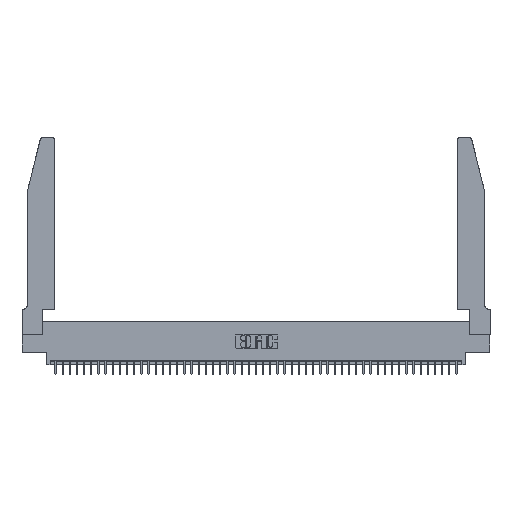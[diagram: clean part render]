
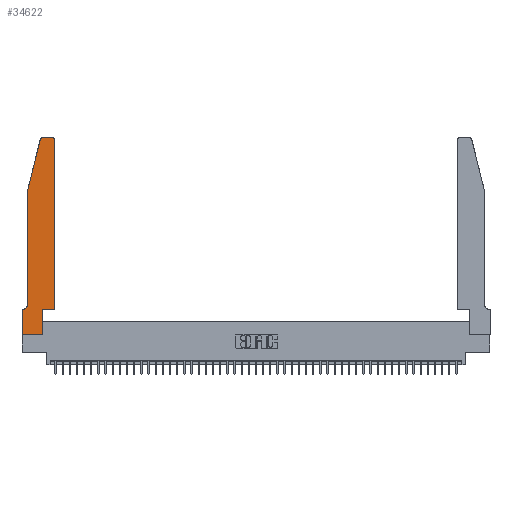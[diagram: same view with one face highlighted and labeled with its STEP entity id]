
A CAD part, top view. The second image highlights one B-rep face of the part: STEP entity #34622.
In plain terms, the highlighted planar face has unit normal (0, 0, 1).
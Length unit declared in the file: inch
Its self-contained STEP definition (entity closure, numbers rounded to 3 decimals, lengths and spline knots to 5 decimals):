
#530 = CARTESIAN_POINT ( 'NONE',  ( 0., 0.35, 0.37 ) ) ;
#876 = VERTEX_POINT ( 'NONE', #14309 ) ;
#877 = DIRECTION ( 'NONE',  ( 0., 1., 0. ) ) ;
#885 = ORIENTED_EDGE ( 'NONE', *, *, #32314, .T. ) ;
#1425 = CARTESIAN_POINT ( 'NONE',  ( 0.0755, 2., 0.37 ) ) ;
#1626 = DIRECTION ( 'NONE',  ( 1., 0., 0. ) ) ;
#1682 = CARTESIAN_POINT ( 'NONE',  ( 0.0755, 2., 0.37 ) ) ;
#1829 = ORIENTED_EDGE ( 'NONE', *, *, #39078, .T. ) ;
#3073 = VERTEX_POINT ( 'NONE', #26422 ) ;
#3277 = VECTOR ( 'NONE', #16940, 39.37008 ) ;
#4284 = CARTESIAN_POINT ( 'NONE',  ( 0.4505, 0.35, 0.37 ) ) ;
#4402 = CARTESIAN_POINT ( 'NONE',  ( 0., 0.35, 0.37 ) ) ;
#5119 = FACE_OUTER_BOUND ( 'NONE', #25854, .T. ) ;
#5715 = VECTOR ( 'NONE', #12567, 39.37008 ) ;
#6719 = CIRCLE ( 'NONE', #35302, 0.03 ) ;
#7092 = CARTESIAN_POINT ( 'NONE',  ( 0.0755, 2., 0.37 ) ) ;
#8177 = LINE ( 'NONE', #20017, #19759 ) ;
#8626 = VERTEX_POINT ( 'NONE', #4402 ) ;
#9294 = DIRECTION ( 'NONE',  ( 0., 0., -1. ) ) ;
#9914 = ORIENTED_EDGE ( 'NONE', *, *, #16836, .T. ) ;
#10335 = EDGE_CURVE ( 'NONE', #876, #18794, #32189, .T. ) ;
#11644 = DIRECTION ( 'NONE',  ( 0., 0., 1. ) ) ;
#12073 = LINE ( 'NONE', #1425, #34520 ) ;
#12094 = CARTESIAN_POINT ( 'NONE',  ( 0.284, 2.72, 0.37 ) ) ;
#12276 = CARTESIAN_POINT ( 'NONE',  ( 0., 0., 0.37 ) ) ;
#12287 = DIRECTION ( 'NONE',  ( -1., 0., 0. ) ) ;
#12304 = VECTOR ( 'NONE', #46153, 39.37008 ) ;
#12517 = EDGE_CURVE ( 'NONE', #29096, #876, #42224, .T. ) ;
#12567 = DIRECTION ( 'NONE',  ( 0., -1., 0. ) ) ;
#12723 = AXIS2_PLACEMENT_3D ( 'NONE', #530, #11644, #40884 ) ;
#13510 = ORIENTED_EDGE ( 'NONE', *, *, #24094, .T. ) ;
#14000 = VERTEX_POINT ( 'NONE', #24568 ) ;
#14307 = CARTESIAN_POINT ( 'NONE',  ( 0.284, 2.75, 0.37 ) ) ;
#14309 = CARTESIAN_POINT ( 'NONE',  ( 0.2865, 0., 0.37 ) ) ;
#14601 = VECTOR ( 'NONE', #1626, 39.37008 ) ;
#16037 = VERTEX_POINT ( 'NONE', #7092 ) ;
#16511 = EDGE_CURVE ( 'NONE', #24232, #22192, #29640, .T. ) ;
#16659 = EDGE_CURVE ( 'NONE', #16037, #28725, #23947, .T. ) ;
#16691 = CARTESIAN_POINT ( 'NONE',  ( 0.0755, 0.35, 0.37 ) ) ;
#16836 = EDGE_CURVE ( 'NONE', #3073, #24232, #8177, .T. ) ;
#16893 = ORIENTED_EDGE ( 'NONE', *, *, #40019, .T. ) ;
#16940 = DIRECTION ( 'NONE',  ( -1., 0., 0. ) ) ;
#17943 = ORIENTED_EDGE ( 'NONE', *, *, #25159, .T. ) ;
#18794 = VERTEX_POINT ( 'NONE', #36374 ) ;
#18908 = PLANE ( 'NONE',  #12723 ) ;
#19759 = VECTOR ( 'NONE', #12287, 39.37008 ) ;
#20017 = CARTESIAN_POINT ( 'NONE',  ( 0.2605, 2.75, 0.37 ) ) ;
#20772 = CARTESIAN_POINT ( 'NONE',  ( 0.4205, 2.72, 0.37 ) ) ;
#20797 = ORIENTED_EDGE ( 'NONE', *, *, #16511, .T. ) ;
#21794 = DIRECTION ( 'NONE',  ( 0., -1., 0. ) ) ;
#22192 = VERTEX_POINT ( 'NONE', #42148 ) ;
#22256 = DIRECTION ( 'NONE',  ( 0., 0., 1. ) ) ;
#23797 = DIRECTION ( 'NONE',  ( -1., 0., 0. ) ) ;
#23947 = LINE ( 'NONE', #1682, #5715 ) ;
#24094 = EDGE_CURVE ( 'NONE', #8626, #29096, #24942, .T. ) ;
#24232 = VERTEX_POINT ( 'NONE', #14307 ) ;
#24389 = CARTESIAN_POINT ( 'NONE',  ( 0.4505, 0.35, 0.37 ) ) ;
#24568 = CARTESIAN_POINT ( 'NONE',  ( 0.0055, 0.35, 0.37 ) ) ;
#24851 = DIRECTION ( 'NONE',  ( 0., 0., 1. ) ) ;
#24919 = LINE ( 'NONE', #34840, #12304 ) ;
#24942 = LINE ( 'NONE', #33136, #25569 ) ;
#25159 = EDGE_CURVE ( 'NONE', #14000, #8626, #35069, .T. ) ;
#25569 = VECTOR ( 'NONE', #21794, 39.37008 ) ;
#25854 = EDGE_LOOP ( 'NONE', ( #9914, #20797, #1829, #39049, #16893, #17943, #13510, #46737, #29060, #43255, #885, #42871 ) ) ;
#26422 = CARTESIAN_POINT ( 'NONE',  ( 0.4205, 2.75, 0.37 ) ) ;
#28725 = VERTEX_POINT ( 'NONE', #36378 ) ;
#29060 = ORIENTED_EDGE ( 'NONE', *, *, #10335, .T. ) ;
#29096 = VERTEX_POINT ( 'NONE', #43020 ) ;
#29640 = CIRCLE ( 'NONE', #39672, 0.03 ) ;
#29768 = VECTOR ( 'NONE', #35822, 39.37008 ) ;
#32189 = LINE ( 'NONE', #36060, #29768 ) ;
#32314 = EDGE_CURVE ( 'NONE', #33525, #44101, #34249, .T. ) ;
#33136 = CARTESIAN_POINT ( 'NONE',  ( 0., 0., 0.37 ) ) ;
#33417 = VECTOR ( 'NONE', #877, 39.37008 ) ;
#33525 = VERTEX_POINT ( 'NONE', #24389 ) ;
#34249 = LINE ( 'NONE', #4284, #33417 ) ;
#34520 = VECTOR ( 'NONE', #37447, 39.37008 ) ;
#34589 = CIRCLE ( 'NONE', #35373, 0.07 ) ;
#34622 = ADVANCED_FACE ( 'NONE', ( #5119 ), #18908, .T. ) ;
#34840 = CARTESIAN_POINT ( 'NONE',  ( 0.4505, 0.35, 0.37 ) ) ;
#35069 = LINE ( 'NONE', #16691, #3277 ) ;
#35302 = AXIS2_PLACEMENT_3D ( 'NONE', #20772, #24851, #35985 ) ;
#35373 = AXIS2_PLACEMENT_3D ( 'NONE', #35396, #9294, #23797 ) ;
#35396 = CARTESIAN_POINT ( 'NONE',  ( 0.0055, 0.42, 0.37 ) ) ;
#35822 = DIRECTION ( 'NONE',  ( 0., 1., 0. ) ) ;
#35985 = DIRECTION ( 'NONE',  ( 1., 0., 0. ) ) ;
#36060 = CARTESIAN_POINT ( 'NONE',  ( 0.2865, 0.35, 0.37 ) ) ;
#36374 = CARTESIAN_POINT ( 'NONE',  ( 0.2865, 0.35, 0.37 ) ) ;
#36378 = CARTESIAN_POINT ( 'NONE',  ( 0.0755, 0.42, 0.37 ) ) ;
#37224 = DIRECTION ( 'NONE',  ( 1., 0., 0. ) ) ;
#37447 = DIRECTION ( 'NONE',  ( -0.239, -0.971, 0. ) ) ;
#39049 = ORIENTED_EDGE ( 'NONE', *, *, #16659, .T. ) ;
#39078 = EDGE_CURVE ( 'NONE', #22192, #16037, #12073, .T. ) ;
#39129 = EDGE_CURVE ( 'NONE', #44101, #3073, #6719, .T. ) ;
#39672 = AXIS2_PLACEMENT_3D ( 'NONE', #12094, #22256, #37224 ) ;
#40019 = EDGE_CURVE ( 'NONE', #28725, #14000, #34589, .T. ) ;
#40884 = DIRECTION ( 'NONE',  ( 1., 0., 0. ) ) ;
#41713 = EDGE_CURVE ( 'NONE', #18794, #33525, #24919, .T. ) ;
#42148 = CARTESIAN_POINT ( 'NONE',  ( 0.25487, 2.72718, 0.37 ) ) ;
#42224 = LINE ( 'NONE', #12276, #14601 ) ;
#42871 = ORIENTED_EDGE ( 'NONE', *, *, #39129, .T. ) ;
#43020 = CARTESIAN_POINT ( 'NONE',  ( 0., 0., 0.37 ) ) ;
#43255 = ORIENTED_EDGE ( 'NONE', *, *, #41713, .T. ) ;
#43393 = CARTESIAN_POINT ( 'NONE',  ( 0.4505, 2.72, 0.37 ) ) ;
#44101 = VERTEX_POINT ( 'NONE', #43393 ) ;
#46153 = DIRECTION ( 'NONE',  ( 1., 0., 0. ) ) ;
#46737 = ORIENTED_EDGE ( 'NONE', *, *, #12517, .T. ) ;
